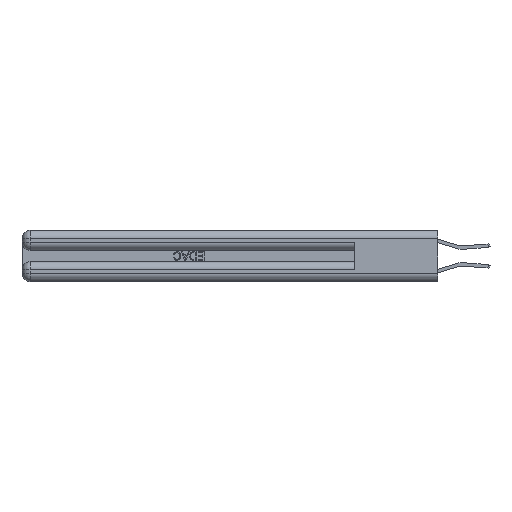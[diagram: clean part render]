
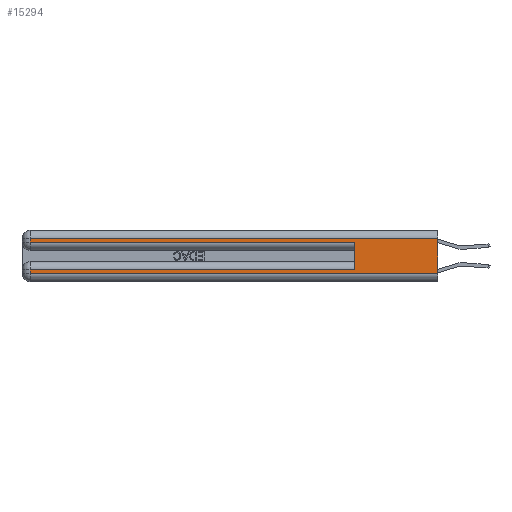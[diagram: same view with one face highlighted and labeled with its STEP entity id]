
A CAD part, left-side view. The second image highlights one B-rep face of the part: STEP entity #15294.
In plain terms, the highlighted planar face has unit normal (-1, 0, 0).
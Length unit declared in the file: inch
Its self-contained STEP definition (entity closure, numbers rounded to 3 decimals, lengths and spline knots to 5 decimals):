
#155 = DIRECTION ( 'NONE',  ( 0., 0., 1. ) ) ;
#507 = PLANE ( 'NONE',  #15337 ) ;
#656 = VECTOR ( 'NONE', #1443, 39.37008 ) ;
#675 = VECTOR ( 'NONE', #7105, 39.37008 ) ;
#868 = DIRECTION ( 'NONE',  ( 0., 0., -1. ) ) ;
#1109 = ORIENTED_EDGE ( 'NONE', *, *, #16076, .T. ) ;
#1215 = LINE ( 'NONE', #34797, #675 ) ;
#1443 = DIRECTION ( 'NONE',  ( 0., 0., -1. ) ) ;
#2138 = DIRECTION ( 'NONE',  ( 0., 0., -1. ) ) ;
#3563 = LINE ( 'NONE', #17514, #22971 ) ;
#4645 = CARTESIAN_POINT ( 'NONE',  ( 0., 0., 0.06 ) ) ;
#4960 = CARTESIAN_POINT ( 'NONE',  ( 0., 0., 0.31 ) ) ;
#5500 = DIRECTION ( 'NONE',  ( 0., 1., 0. ) ) ;
#7105 = DIRECTION ( 'NONE',  ( 0., -1., 0. ) ) ;
#7254 = VECTOR ( 'NONE', #26177, 39.37008 ) ;
#7372 = LINE ( 'NONE', #9957, #19419 ) ;
#7434 = VERTEX_POINT ( 'NONE', #34438 ) ;
#7476 = EDGE_CURVE ( 'NONE', #12581, #11937, #1215, .T. ) ;
#7891 = EDGE_LOOP ( 'NONE', ( #33385, #33742, #33146, #33130, #17983, #1109, #11367, #30774 ) ) ;
#8213 = LINE ( 'NONE', #18857, #18099 ) ;
#8416 = EDGE_CURVE ( 'NONE', #13476, #12581, #7372, .T. ) ;
#9885 = EDGE_CURVE ( 'NONE', #13860, #35924, #8213, .T. ) ;
#9941 = CARTESIAN_POINT ( 'NONE',  ( 0., 0.6, 0.085 ) ) ;
#9957 = CARTESIAN_POINT ( 'NONE',  ( 0., 2.94, 0.37 ) ) ;
#10081 = CARTESIAN_POINT ( 'NONE',  ( 0., 0., 0.37 ) ) ;
#10710 = EDGE_CURVE ( 'NONE', #19890, #13860, #30090, .T. ) ;
#10880 = CARTESIAN_POINT ( 'NONE',  ( 0., 0., 0.31 ) ) ;
#11367 = ORIENTED_EDGE ( 'NONE', *, *, #8416, .T. ) ;
#11537 = FACE_OUTER_BOUND ( 'NONE', #7891, .T. ) ;
#11937 = VERTEX_POINT ( 'NONE', #4645 ) ;
#11989 = DIRECTION ( 'NONE',  ( 0., 1., 0. ) ) ;
#12581 = VERTEX_POINT ( 'NONE', #34238 ) ;
#13476 = VERTEX_POINT ( 'NONE', #24746 ) ;
#13860 = VERTEX_POINT ( 'NONE', #18718 ) ;
#15294 = ADVANCED_FACE ( 'NONE', ( #11537 ), #507, .F. ) ;
#15337 = AXIS2_PLACEMENT_3D ( 'NONE', #33912, #34267, #868 ) ;
#16076 = EDGE_CURVE ( 'NONE', #32398, #13476, #3563, .T. ) ;
#17514 = CARTESIAN_POINT ( 'NONE',  ( 0., 0., 0.085 ) ) ;
#17940 = LINE ( 'NONE', #35457, #7254 ) ;
#17983 = ORIENTED_EDGE ( 'NONE', *, *, #25751, .F. ) ;
#18099 = VECTOR ( 'NONE', #2138, 39.37008 ) ;
#18569 = DIRECTION ( 'NONE',  ( 0., 0., -1. ) ) ;
#18718 = CARTESIAN_POINT ( 'NONE',  ( 0., 2.94, 0.31 ) ) ;
#18857 = CARTESIAN_POINT ( 'NONE',  ( 0., 2.94, 0.37 ) ) ;
#19419 = VECTOR ( 'NONE', #18569, 39.37008 ) ;
#19702 = EDGE_CURVE ( 'NONE', #35924, #7434, #17940, .T. ) ;
#19890 = VERTEX_POINT ( 'NONE', #10880 ) ;
#22971 = VECTOR ( 'NONE', #11989, 39.37008 ) ;
#24331 = EDGE_CURVE ( 'NONE', #19890, #11937, #35200, .T. ) ;
#24746 = CARTESIAN_POINT ( 'NONE',  ( 0., 2.94, 0.085 ) ) ;
#25751 = EDGE_CURVE ( 'NONE', #32398, #7434, #36127, .T. ) ;
#26177 = DIRECTION ( 'NONE',  ( 0., -1., 0. ) ) ;
#27503 = VECTOR ( 'NONE', #5500, 39.37008 ) ;
#30090 = LINE ( 'NONE', #4960, #27503 ) ;
#30284 = CARTESIAN_POINT ( 'NONE',  ( 0., 0.6, 0.145 ) ) ;
#30774 = ORIENTED_EDGE ( 'NONE', *, *, #7476, .T. ) ;
#32398 = VERTEX_POINT ( 'NONE', #9941 ) ;
#33022 = CARTESIAN_POINT ( 'NONE',  ( 0., 2.94, 0.285 ) ) ;
#33130 = ORIENTED_EDGE ( 'NONE', *, *, #19702, .T. ) ;
#33146 = ORIENTED_EDGE ( 'NONE', *, *, #9885, .T. ) ;
#33385 = ORIENTED_EDGE ( 'NONE', *, *, #24331, .F. ) ;
#33742 = ORIENTED_EDGE ( 'NONE', *, *, #10710, .T. ) ;
#33912 = CARTESIAN_POINT ( 'NONE',  ( 0., 0., 0.37 ) ) ;
#34238 = CARTESIAN_POINT ( 'NONE',  ( 0., 2.94, 0.06 ) ) ;
#34267 = DIRECTION ( 'NONE',  ( 1., 0., 0. ) ) ;
#34438 = CARTESIAN_POINT ( 'NONE',  ( 0., 0.6, 0.285 ) ) ;
#34797 = CARTESIAN_POINT ( 'NONE',  ( 0., 0., 0.06 ) ) ;
#35200 = LINE ( 'NONE', #10081, #656 ) ;
#35281 = VECTOR ( 'NONE', #155, 39.37008 ) ;
#35457 = CARTESIAN_POINT ( 'NONE',  ( 0., 0., 0.285 ) ) ;
#35924 = VERTEX_POINT ( 'NONE', #33022 ) ;
#36127 = LINE ( 'NONE', #30284, #35281 ) ;
